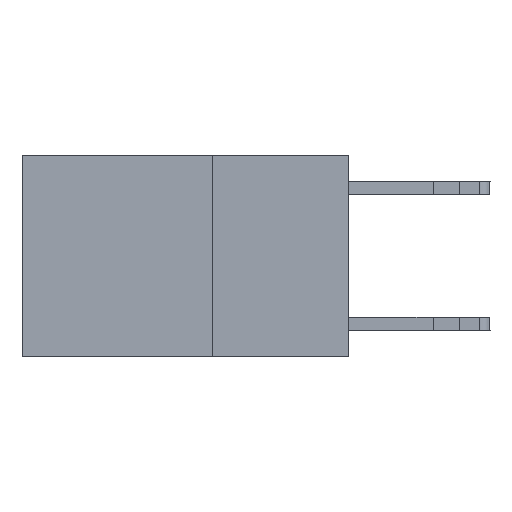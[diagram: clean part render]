
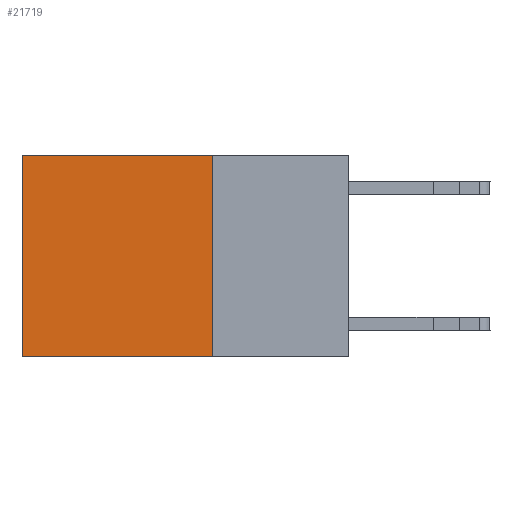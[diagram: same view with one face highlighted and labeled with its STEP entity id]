
A CAD part, left-side view. The second image highlights one B-rep face of the part: STEP entity #21719.
In plain terms, the highlighted planar face has unit normal (-1, 0, 0).
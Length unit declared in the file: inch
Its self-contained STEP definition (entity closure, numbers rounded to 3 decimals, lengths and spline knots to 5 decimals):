
#1343 = EDGE_CURVE ( 'NONE', #14894, #23841, #10793, .T. ) ;
#1410 = DIRECTION ( 'NONE',  ( 0., 1., 0. ) ) ;
#1556 = EDGE_CURVE ( 'NONE', #18105, #14894, #16769, .T. ) ;
#2744 = VERTEX_POINT ( 'NONE', #21525 ) ;
#2833 = EDGE_LOOP ( 'NONE', ( #23660, #17644, #11554, #3526 ) ) ;
#3385 = VECTOR ( 'NONE', #17026, 39.37008 ) ;
#3526 = ORIENTED_EDGE ( 'NONE', *, *, #1556, .T. ) ;
#4035 = CARTESIAN_POINT ( 'NONE',  ( 0.2625, 0.6, -0.37 ) ) ;
#4578 = DIRECTION ( 'NONE',  ( 0., 0., -1. ) ) ;
#4808 = CARTESIAN_POINT ( 'NONE',  ( 0.2625, 0.6, 0. ) ) ;
#6322 = EDGE_CURVE ( 'NONE', #2744, #23841, #17199, .T. ) ;
#6394 = EDGE_CURVE ( 'NONE', #18105, #2744, #10911, .T. ) ;
#8253 = CARTESIAN_POINT ( 'NONE',  ( 0.2625, 0.25, 0. ) ) ;
#8651 = FACE_OUTER_BOUND ( 'NONE', #2833, .T. ) ;
#10434 = DIRECTION ( 'NONE',  ( 0., 0., -1. ) ) ;
#10688 = CARTESIAN_POINT ( 'NONE',  ( 0.2625, 0.25, 0. ) ) ;
#10793 = LINE ( 'NONE', #4808, #24267 ) ;
#10911 = LINE ( 'NONE', #17017, #18136 ) ;
#11554 = ORIENTED_EDGE ( 'NONE', *, *, #6394, .F. ) ;
#12811 = DIRECTION ( 'NONE',  ( 0., 0., -1. ) ) ;
#14257 = PLANE ( 'NONE',  #23118 ) ;
#14894 = VERTEX_POINT ( 'NONE', #21167 ) ;
#15162 = CARTESIAN_POINT ( 'NONE',  ( 0.2625, 0.25, -0.37 ) ) ;
#16769 = LINE ( 'NONE', #17157, #3385 ) ;
#17017 = CARTESIAN_POINT ( 'NONE',  ( 0.2625, 0.25, 0. ) ) ;
#17026 = DIRECTION ( 'NONE',  ( 0., 1., 0. ) ) ;
#17157 = CARTESIAN_POINT ( 'NONE',  ( 0.2625, 0.25, 0. ) ) ;
#17199 = LINE ( 'NONE', #15162, #23459 ) ;
#17644 = ORIENTED_EDGE ( 'NONE', *, *, #6322, .F. ) ;
#18105 = VERTEX_POINT ( 'NONE', #8253 ) ;
#18136 = VECTOR ( 'NONE', #12811, 39.37008 ) ;
#21167 = CARTESIAN_POINT ( 'NONE',  ( 0.2625, 0.6, 0. ) ) ;
#21525 = CARTESIAN_POINT ( 'NONE',  ( 0.2625, 0.25, -0.37 ) ) ;
#21719 = ADVANCED_FACE ( 'NONE', ( #8651 ), #14257, .F. ) ;
#22046 = DIRECTION ( 'NONE',  ( 1., 0., 0. ) ) ;
#23118 = AXIS2_PLACEMENT_3D ( 'NONE', #10688, #22046, #4578 ) ;
#23459 = VECTOR ( 'NONE', #1410, 39.37008 ) ;
#23660 = ORIENTED_EDGE ( 'NONE', *, *, #1343, .T. ) ;
#23841 = VERTEX_POINT ( 'NONE', #4035 ) ;
#24267 = VECTOR ( 'NONE', #10434, 39.37008 ) ;
